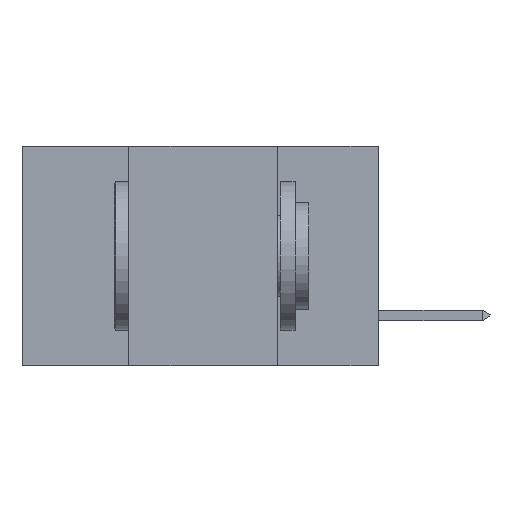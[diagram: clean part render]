
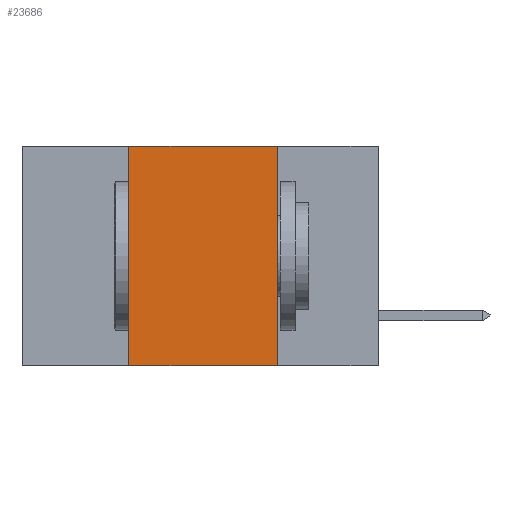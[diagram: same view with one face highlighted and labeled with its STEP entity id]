
A CAD part, left-side view. The second image highlights one B-rep face of the part: STEP entity #23686.
In plain terms, the highlighted planar face has unit normal (-1, 0, 0).
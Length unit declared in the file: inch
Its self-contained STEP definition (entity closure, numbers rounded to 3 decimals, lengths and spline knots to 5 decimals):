
#326 = ORIENTED_EDGE ( 'NONE', *, *, #865, .F. ) ;
#865 = EDGE_CURVE ( 'NONE', #25019, #16604, #2590, .T. ) ;
#1350 = CARTESIAN_POINT ( 'NONE',  ( 0., 0.42, 0. ) ) ;
#1784 = PLANE ( 'NONE',  #14923 ) ;
#2590 = LINE ( 'NONE', #2733, #9149 ) ;
#2591 = ORIENTED_EDGE ( 'NONE', *, *, #16047, .F. ) ;
#2733 = CARTESIAN_POINT ( 'NONE',  ( 0., 0.6, 0. ) ) ;
#4594 = DIRECTION ( 'NONE',  ( 1., 0., 0. ) ) ;
#6357 = LINE ( 'NONE', #22281, #19341 ) ;
#6433 = CARTESIAN_POINT ( 'NONE',  ( 0., 0.17, 0. ) ) ;
#7133 = DIRECTION ( 'NONE',  ( 0., 0., -1. ) ) ;
#7515 = DIRECTION ( 'NONE',  ( 0., 0., -1. ) ) ;
#9149 = VECTOR ( 'NONE', #22727, 39.37008 ) ;
#10276 = CARTESIAN_POINT ( 'NONE',  ( 0., 0.42, -0.37 ) ) ;
#11647 = FACE_OUTER_BOUND ( 'NONE', #18145, .T. ) ;
#14782 = EDGE_CURVE ( 'NONE', #21722, #15638, #6357, .T. ) ;
#14923 = AXIS2_PLACEMENT_3D ( 'NONE', #16302, #4594, #7133 ) ;
#15006 = CARTESIAN_POINT ( 'NONE',  ( 0., 0.17, -0.37 ) ) ;
#15638 = VERTEX_POINT ( 'NONE', #15006 ) ;
#16047 = EDGE_CURVE ( 'NONE', #21722, #25019, #24043, .T. ) ;
#16100 = VECTOR ( 'NONE', #21485, 39.37008 ) ;
#16302 = CARTESIAN_POINT ( 'NONE',  ( 0., 0.6, 0. ) ) ;
#16604 = VERTEX_POINT ( 'NONE', #6433 ) ;
#17578 = ORIENTED_EDGE ( 'NONE', *, *, #14782, .T. ) ;
#18145 = EDGE_LOOP ( 'NONE', ( #25885, #326, #2591, #17578 ) ) ;
#18300 = CARTESIAN_POINT ( 'NONE',  ( 0., 0.42, 0. ) ) ;
#18717 = VECTOR ( 'NONE', #7515, 39.37008 ) ;
#19082 = CARTESIAN_POINT ( 'NONE',  ( 0., 0.17, 0. ) ) ;
#19341 = VECTOR ( 'NONE', #24082, 39.37008 ) ;
#21485 = DIRECTION ( 'NONE',  ( 0., 0., 1. ) ) ;
#21722 = VERTEX_POINT ( 'NONE', #10276 ) ;
#22281 = CARTESIAN_POINT ( 'NONE',  ( 0., 0.6, -0.37 ) ) ;
#22536 = EDGE_CURVE ( 'NONE', #16604, #15638, #25844, .T. ) ;
#22727 = DIRECTION ( 'NONE',  ( 0., -1., 0. ) ) ;
#23686 = ADVANCED_FACE ( 'NONE', ( #11647 ), #1784, .F. ) ;
#24043 = LINE ( 'NONE', #1350, #16100 ) ;
#24082 = DIRECTION ( 'NONE',  ( 0., -1., 0. ) ) ;
#25019 = VERTEX_POINT ( 'NONE', #18300 ) ;
#25844 = LINE ( 'NONE', #19082, #18717 ) ;
#25885 = ORIENTED_EDGE ( 'NONE', *, *, #22536, .F. ) ;
